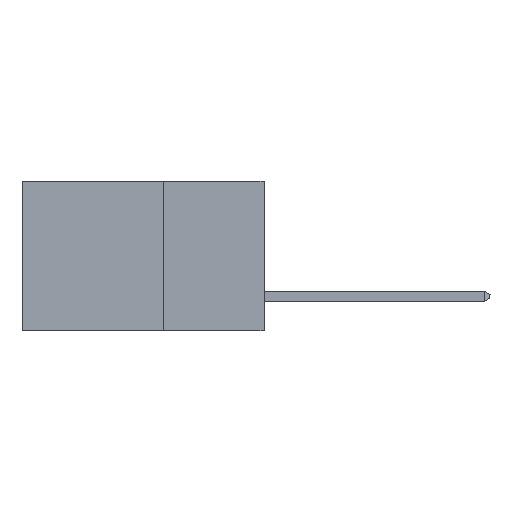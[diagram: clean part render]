
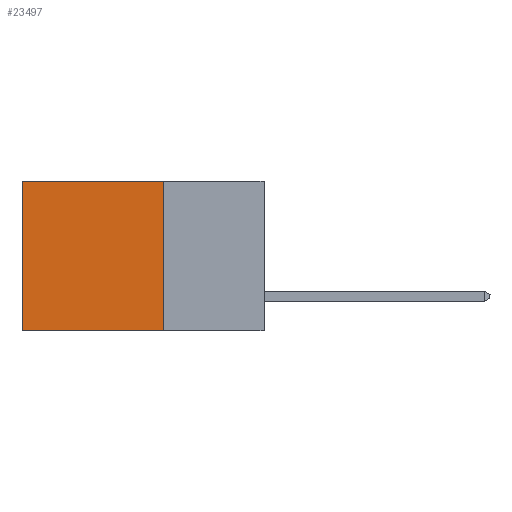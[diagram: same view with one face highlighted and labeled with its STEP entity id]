
A CAD part, left-side view. The second image highlights one B-rep face of the part: STEP entity #23497.
In plain terms, the highlighted planar face has unit normal (-1, 0, 0).
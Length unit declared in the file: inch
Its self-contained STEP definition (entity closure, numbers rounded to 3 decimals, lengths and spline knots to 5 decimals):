
#685 = CARTESIAN_POINT ( 'NONE',  ( 0.298, 0.25, 0. ) ) ;
#967 = DIRECTION ( 'NONE',  ( 0., 0., -1. ) ) ;
#1045 = VECTOR ( 'NONE', #13826, 39.37008 ) ;
#1333 = LINE ( 'NONE', #29891, #5440 ) ;
#1865 = CARTESIAN_POINT ( 'NONE',  ( 0.298, 0.6, -0.37 ) ) ;
#2684 = VECTOR ( 'NONE', #10585, 39.37008 ) ;
#4299 = VERTEX_POINT ( 'NONE', #4335 ) ;
#4335 = CARTESIAN_POINT ( 'NONE',  ( 0.298, 0.6, 0. ) ) ;
#4693 = EDGE_CURVE ( 'NONE', #30106, #5655, #1333, .T. ) ;
#5440 = VECTOR ( 'NONE', #967, 39.37008 ) ;
#5655 = VERTEX_POINT ( 'NONE', #11948 ) ;
#5954 = PLANE ( 'NONE',  #27817 ) ;
#7876 = FACE_OUTER_BOUND ( 'NONE', #24961, .T. ) ;
#9111 = EDGE_CURVE ( 'NONE', #4299, #11036, #14638, .T. ) ;
#10585 = DIRECTION ( 'NONE',  ( 0., 1., 0. ) ) ;
#11036 = VERTEX_POINT ( 'NONE', #1865 ) ;
#11066 = CARTESIAN_POINT ( 'NONE',  ( 0.298, 0.6, 0. ) ) ;
#11948 = CARTESIAN_POINT ( 'NONE',  ( 0.298, 0.25, -0.37 ) ) ;
#13052 = CARTESIAN_POINT ( 'NONE',  ( 0.298, 0.25, 0. ) ) ;
#13696 = ORIENTED_EDGE ( 'NONE', *, *, #4693, .F. ) ;
#13826 = DIRECTION ( 'NONE',  ( 0., 0., -1. ) ) ;
#14638 = LINE ( 'NONE', #11066, #1045 ) ;
#14807 = EDGE_CURVE ( 'NONE', #30106, #4299, #28676, .T. ) ;
#14885 = EDGE_CURVE ( 'NONE', #5655, #11036, #26088, .T. ) ;
#16624 = VECTOR ( 'NONE', #20304, 39.37008 ) ;
#18013 = ORIENTED_EDGE ( 'NONE', *, *, #14885, .F. ) ;
#18121 = DIRECTION ( 'NONE',  ( 1., 0., 0. ) ) ;
#18482 = CARTESIAN_POINT ( 'NONE',  ( 0.298, 0.25, 0. ) ) ;
#18911 = ORIENTED_EDGE ( 'NONE', *, *, #14807, .T. ) ;
#20304 = DIRECTION ( 'NONE',  ( 0., 1., 0. ) ) ;
#22387 = CARTESIAN_POINT ( 'NONE',  ( 0.298, 0.25, -0.37 ) ) ;
#22840 = DIRECTION ( 'NONE',  ( 0., 0., -1. ) ) ;
#23497 = ADVANCED_FACE ( 'NONE', ( #7876 ), #5954, .F. ) ;
#24865 = ORIENTED_EDGE ( 'NONE', *, *, #9111, .T. ) ;
#24961 = EDGE_LOOP ( 'NONE', ( #24865, #18013, #13696, #18911 ) ) ;
#26088 = LINE ( 'NONE', #22387, #2684 ) ;
#27817 = AXIS2_PLACEMENT_3D ( 'NONE', #13052, #18121, #22840 ) ;
#28676 = LINE ( 'NONE', #685, #16624 ) ;
#29891 = CARTESIAN_POINT ( 'NONE',  ( 0.298, 0.25, 0. ) ) ;
#30106 = VERTEX_POINT ( 'NONE', #18482 ) ;
